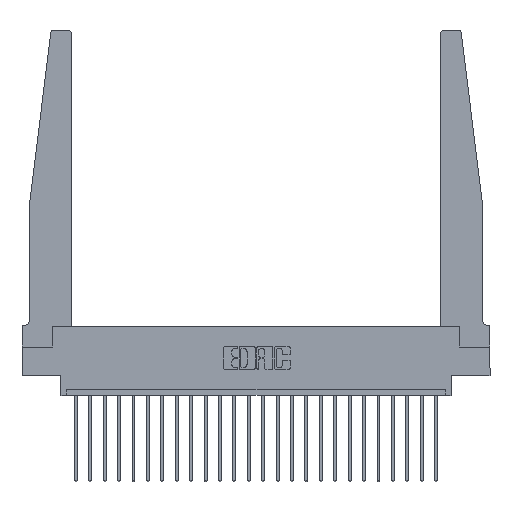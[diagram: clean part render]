
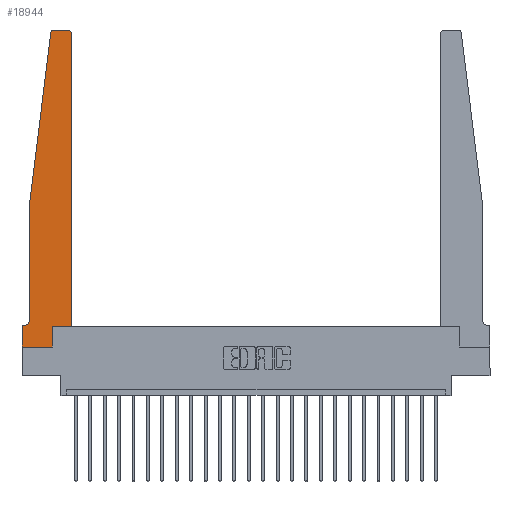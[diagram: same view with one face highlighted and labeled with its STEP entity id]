
A CAD part, top view. The second image highlights one B-rep face of the part: STEP entity #18944.
In plain terms, the highlighted planar face has unit normal (0, 0, 1).
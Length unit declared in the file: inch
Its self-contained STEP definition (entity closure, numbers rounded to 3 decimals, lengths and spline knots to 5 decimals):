
#137 = CARTESIAN_POINT ( 'NONE',  ( 0.425, 0.18, 0.37 ) ) ;
#181 = CARTESIAN_POINT ( 'NONE',  ( 0.2605, 0.18, 0.37 ) ) ;
#301 = DIRECTION ( 'NONE',  ( 1., 0., 0. ) ) ;
#422 = EDGE_CURVE ( 'NONE', #6987, #1725, #16116, .T. ) ;
#492 = ORIENTED_EDGE ( 'NONE', *, *, #5895, .T. ) ;
#774 = LINE ( 'NONE', #10059, #19987 ) ;
#1300 = DIRECTION ( 'NONE',  ( 0., 1., 0. ) ) ;
#1324 = LINE ( 'NONE', #4579, #8003 ) ;
#1396 = ORIENTED_EDGE ( 'NONE', *, *, #18623, .T. ) ;
#1593 = CARTESIAN_POINT ( 'NONE',  ( 0.395, 2.75, 0.37 ) ) ;
#1725 = VERTEX_POINT ( 'NONE', #20978 ) ;
#2113 = CARTESIAN_POINT ( 'NONE',  ( 0.065, 1.25, 0.37 ) ) ;
#2247 = CARTESIAN_POINT ( 'NONE',  ( 0.27653, 2.72, 0.37 ) ) ;
#2309 = ORIENTED_EDGE ( 'NONE', *, *, #5857, .T. ) ;
#2442 = VERTEX_POINT ( 'NONE', #3480 ) ;
#2493 = EDGE_LOOP ( 'NONE', ( #4746, #3567, #492, #21719, #9979, #6207, #20098, #2309, #20929, #21688, #1396, #13767 ) ) ;
#2941 = CARTESIAN_POINT ( 'NONE',  ( 0.395, 2.72, 0.37 ) ) ;
#3100 = CARTESIAN_POINT ( 'NONE',  ( 0.24675, 2.72367, 0.37 ) ) ;
#3401 = DIRECTION ( 'NONE',  ( 1., 0., 0. ) ) ;
#3480 = CARTESIAN_POINT ( 'NONE',  ( 0.425, 0.18, 0.37 ) ) ;
#3567 = ORIENTED_EDGE ( 'NONE', *, *, #11281, .T. ) ;
#3813 = DIRECTION ( 'NONE',  ( 0., -1., 0. ) ) ;
#4178 = EDGE_CURVE ( 'NONE', #10623, #4913, #15674, .T. ) ;
#4579 = CARTESIAN_POINT ( 'NONE',  ( 0.065, 1.25, 0.37 ) ) ;
#4589 = CARTESIAN_POINT ( 'NONE',  ( 0.2605, 0.18, 0.37 ) ) ;
#4734 = DIRECTION ( 'NONE',  ( 0., 0., -1. ) ) ;
#4746 = ORIENTED_EDGE ( 'NONE', *, *, #422, .T. ) ;
#4913 = VERTEX_POINT ( 'NONE', #181 ) ;
#5009 = CARTESIAN_POINT ( 'NONE',  ( 0.25, 2.75, 0.37 ) ) ;
#5634 = CARTESIAN_POINT ( 'NONE',  ( 0., 0., 0.37 ) ) ;
#5677 = EDGE_CURVE ( 'NONE', #20285, #6987, #11170, .T. ) ;
#5834 = DIRECTION ( 'NONE',  ( 0., 0., 1. ) ) ;
#5857 = EDGE_CURVE ( 'NONE', #11857, #10623, #20397, .T. ) ;
#5895 = EDGE_CURVE ( 'NONE', #17477, #11127, #19277, .T. ) ;
#5938 = VECTOR ( 'NONE', #3813, 39.37008 ) ;
#6207 = ORIENTED_EDGE ( 'NONE', *, *, #15174, .T. ) ;
#6209 = AXIS2_PLACEMENT_3D ( 'NONE', #2941, #22352, #6535 ) ;
#6453 = DIRECTION ( 'NONE',  ( 0., -1., 0. ) ) ;
#6535 = DIRECTION ( 'NONE',  ( 1., 0., 0. ) ) ;
#6868 = DIRECTION ( 'NONE',  ( -1., 0., 0. ) ) ;
#6987 = VERTEX_POINT ( 'NONE', #1593 ) ;
#7057 = AXIS2_PLACEMENT_3D ( 'NONE', #14208, #16204, #3401 ) ;
#7338 = EDGE_CURVE ( 'NONE', #11127, #21628, #1324, .T. ) ;
#7464 = CARTESIAN_POINT ( 'NONE',  ( 0.425, 2.72, 0.37 ) ) ;
#8003 = VECTOR ( 'NONE', #6453, 39.37008 ) ;
#8516 = AXIS2_PLACEMENT_3D ( 'NONE', #2247, #5834, #301 ) ;
#8664 = VERTEX_POINT ( 'NONE', #20468 ) ;
#8951 = DIRECTION ( 'NONE',  ( 1., 0., 0. ) ) ;
#9230 = DIRECTION ( 'NONE',  ( -0.122, -0.992, 0. ) ) ;
#9807 = CIRCLE ( 'NONE', #8516, 0.03 ) ;
#9979 = ORIENTED_EDGE ( 'NONE', *, *, #11341, .T. ) ;
#10059 = CARTESIAN_POINT ( 'NONE',  ( 0.425, 0.18, 0.37 ) ) ;
#10133 = CARTESIAN_POINT ( 'NONE',  ( 0.015, 0.2375, 0.37 ) ) ;
#10623 = VERTEX_POINT ( 'NONE', #14646 ) ;
#11100 = CARTESIAN_POINT ( 'NONE',  ( 0., 0.1875, 0.37 ) ) ;
#11127 = VERTEX_POINT ( 'NONE', #21503 ) ;
#11170 = CIRCLE ( 'NONE', #6209, 0.03 ) ;
#11198 = CIRCLE ( 'NONE', #17834, 0.05 ) ;
#11281 = EDGE_CURVE ( 'NONE', #1725, #17477, #9807, .T. ) ;
#11319 = VECTOR ( 'NONE', #6868, 39.37008 ) ;
#11341 = EDGE_CURVE ( 'NONE', #21628, #8664, #11198, .T. ) ;
#11424 = VECTOR ( 'NONE', #1300, 39.37008 ) ;
#11574 = EDGE_CURVE ( 'NONE', #4913, #2442, #14876, .T. ) ;
#11857 = VERTEX_POINT ( 'NONE', #13160 ) ;
#12475 = PLANE ( 'NONE',  #7057 ) ;
#12613 = CARTESIAN_POINT ( 'NONE',  ( 0.065, 0.2375, 0.37 ) ) ;
#13160 = CARTESIAN_POINT ( 'NONE',  ( 0., 0., 0.37 ) ) ;
#13767 = ORIENTED_EDGE ( 'NONE', *, *, #5677, .T. ) ;
#14208 = CARTESIAN_POINT ( 'NONE',  ( 0., 0.1875, 0.37 ) ) ;
#14553 = CARTESIAN_POINT ( 'NONE',  ( 0., 0., 0.37 ) ) ;
#14570 = VECTOR ( 'NONE', #9230, 39.37008 ) ;
#14646 = CARTESIAN_POINT ( 'NONE',  ( 0.2605, 0., 0.37 ) ) ;
#14712 = CARTESIAN_POINT ( 'NONE',  ( 0.065, 0.1875, 0.37 ) ) ;
#14876 = LINE ( 'NONE', #137, #22681 ) ;
#14883 = VECTOR ( 'NONE', #19938, 39.37008 ) ;
#15174 = EDGE_CURVE ( 'NONE', #8664, #20333, #20855, .T. ) ;
#15674 = LINE ( 'NONE', #4589, #11424 ) ;
#15752 = LINE ( 'NONE', #14553, #5938 ) ;
#16116 = LINE ( 'NONE', #5009, #11319 ) ;
#16204 = DIRECTION ( 'NONE',  ( 0., 0., 1. ) ) ;
#17255 = EDGE_CURVE ( 'NONE', #20333, #11857, #15752, .T. ) ;
#17477 = VERTEX_POINT ( 'NONE', #3100 ) ;
#17834 = AXIS2_PLACEMENT_3D ( 'NONE', #10133, #4734, #22670 ) ;
#18623 = EDGE_CURVE ( 'NONE', #2442, #20285, #774, .T. ) ;
#18944 = ADVANCED_FACE ( 'NONE', ( #21132 ), #12475, .T. ) ;
#19277 = LINE ( 'NONE', #2113, #14570 ) ;
#19938 = DIRECTION ( 'NONE',  ( 1., 0., 0. ) ) ;
#19987 = VECTOR ( 'NONE', #22599, 39.37008 ) ;
#20013 = VECTOR ( 'NONE', #21448, 39.37008 ) ;
#20098 = ORIENTED_EDGE ( 'NONE', *, *, #17255, .T. ) ;
#20285 = VERTEX_POINT ( 'NONE', #7464 ) ;
#20333 = VERTEX_POINT ( 'NONE', #11100 ) ;
#20397 = LINE ( 'NONE', #5634, #14883 ) ;
#20468 = CARTESIAN_POINT ( 'NONE',  ( 0.015, 0.1875, 0.37 ) ) ;
#20855 = LINE ( 'NONE', #14712, #20013 ) ;
#20929 = ORIENTED_EDGE ( 'NONE', *, *, #4178, .T. ) ;
#20978 = CARTESIAN_POINT ( 'NONE',  ( 0.27653, 2.75, 0.37 ) ) ;
#21132 = FACE_OUTER_BOUND ( 'NONE', #2493, .T. ) ;
#21448 = DIRECTION ( 'NONE',  ( -1., 0., 0. ) ) ;
#21503 = CARTESIAN_POINT ( 'NONE',  ( 0.065, 1.25, 0.37 ) ) ;
#21628 = VERTEX_POINT ( 'NONE', #12613 ) ;
#21688 = ORIENTED_EDGE ( 'NONE', *, *, #11574, .T. ) ;
#21719 = ORIENTED_EDGE ( 'NONE', *, *, #7338, .T. ) ;
#22352 = DIRECTION ( 'NONE',  ( 0., 0., 1. ) ) ;
#22599 = DIRECTION ( 'NONE',  ( 0., 1., 0. ) ) ;
#22670 = DIRECTION ( 'NONE',  ( -1., 0., 0. ) ) ;
#22681 = VECTOR ( 'NONE', #8951, 39.37008 ) ;
